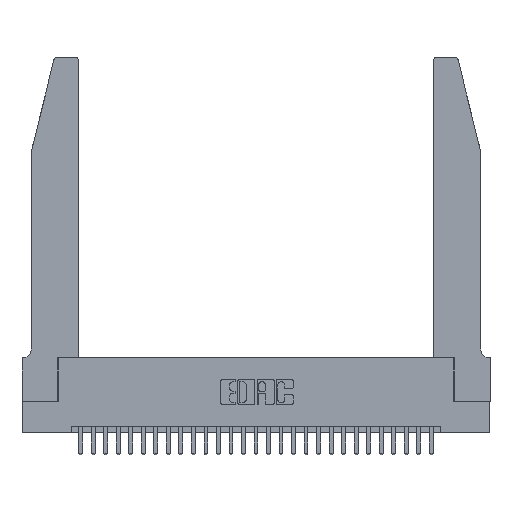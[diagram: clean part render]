
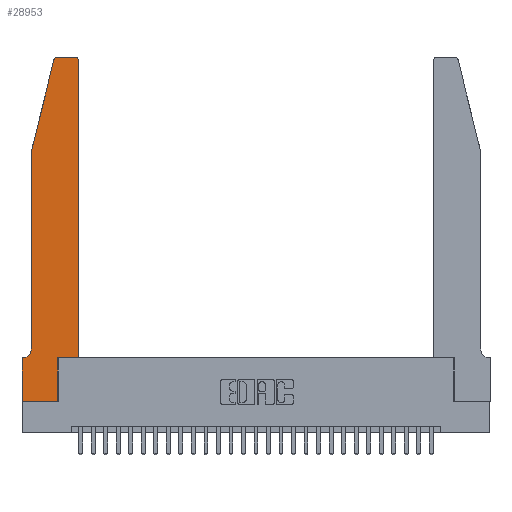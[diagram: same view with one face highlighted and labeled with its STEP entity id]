
A CAD part, top view. The second image highlights one B-rep face of the part: STEP entity #28953.
In plain terms, the highlighted planar face has unit normal (0, 0, 1).
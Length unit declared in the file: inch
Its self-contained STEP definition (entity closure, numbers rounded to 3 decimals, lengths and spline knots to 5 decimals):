
#121 = DIRECTION ( 'NONE',  ( 0., 0., 1. ) ) ;
#394 = VERTEX_POINT ( 'NONE', #3091 ) ;
#399 = ORIENTED_EDGE ( 'NONE', *, *, #19376, .T. ) ;
#493 = CARTESIAN_POINT ( 'NONE',  ( 0.0055, 0.42, 0.37 ) ) ;
#527 = EDGE_CURVE ( 'NONE', #394, #2790, #25859, .T. ) ;
#742 = LINE ( 'NONE', #20856, #5367 ) ;
#2523 = CARTESIAN_POINT ( 'NONE',  ( 0.284, 2.72, 0.37 ) ) ;
#2575 = CARTESIAN_POINT ( 'NONE',  ( 0.2865, 0.35, 0.37 ) ) ;
#2790 = VERTEX_POINT ( 'NONE', #20274 ) ;
#3091 = CARTESIAN_POINT ( 'NONE',  ( 0., 0.35, 0.37 ) ) ;
#3295 = VERTEX_POINT ( 'NONE', #20784 ) ;
#3761 = CARTESIAN_POINT ( 'NONE',  ( 0.4505, 0.35, 0.37 ) ) ;
#4062 = EDGE_CURVE ( 'NONE', #7007, #14862, #15695, .T. ) ;
#4589 = DIRECTION ( 'NONE',  ( 1., 0., 0. ) ) ;
#4986 = DIRECTION ( 'NONE',  ( -0.239, -0.971, 0. ) ) ;
#5217 = FACE_OUTER_BOUND ( 'NONE', #7160, .T. ) ;
#5367 = VECTOR ( 'NONE', #4986, 39.37008 ) ;
#5966 = DIRECTION ( 'NONE',  ( 0., 1., 0. ) ) ;
#6171 = DIRECTION ( 'NONE',  ( -1., 0., 0. ) ) ;
#7007 = VERTEX_POINT ( 'NONE', #2575 ) ;
#7160 = EDGE_LOOP ( 'NONE', ( #26678, #16221, #22059, #18440, #28837, #10267, #23125, #26511, #399, #26267, #19559, #9952 ) ) ;
#7229 = DIRECTION ( 'NONE',  ( 1., 0., 0. ) ) ;
#7350 = CIRCLE ( 'NONE', #19434, 0.07 ) ;
#7730 = VECTOR ( 'NONE', #8560, 39.37008 ) ;
#8003 = EDGE_CURVE ( 'NONE', #13516, #18174, #26152, .T. ) ;
#8112 = DIRECTION ( 'NONE',  ( 0., -1., 0. ) ) ;
#8218 = CARTESIAN_POINT ( 'NONE',  ( 0.4505, 2.72, 0.37 ) ) ;
#8560 = DIRECTION ( 'NONE',  ( 0., -1., 0. ) ) ;
#8812 = LINE ( 'NONE', #11809, #19114 ) ;
#9272 = PLANE ( 'NONE',  #11984 ) ;
#9444 = DIRECTION ( 'NONE',  ( 1., 0., 0. ) ) ;
#9820 = DIRECTION ( 'NONE',  ( 0., 0., -1. ) ) ;
#9952 = ORIENTED_EDGE ( 'NONE', *, *, #8003, .T. ) ;
#10073 = VERTEX_POINT ( 'NONE', #28441 ) ;
#10267 = ORIENTED_EDGE ( 'NONE', *, *, #28495, .T. ) ;
#10675 = AXIS2_PLACEMENT_3D ( 'NONE', #2523, #121, #4589 ) ;
#11598 = VECTOR ( 'NONE', #8112, 39.37008 ) ;
#11687 = DIRECTION ( 'NONE',  ( -1., 0., 0. ) ) ;
#11809 = CARTESIAN_POINT ( 'NONE',  ( 0., 0., 0.37 ) ) ;
#11901 = CARTESIAN_POINT ( 'NONE',  ( 0.4505, 0.35, 0.37 ) ) ;
#11984 = AXIS2_PLACEMENT_3D ( 'NONE', #19643, #15885, #15791 ) ;
#12388 = CARTESIAN_POINT ( 'NONE',  ( 0.0055, 0.35, 0.37 ) ) ;
#13315 = EDGE_CURVE ( 'NONE', #28248, #26819, #25479, .T. ) ;
#13516 = VERTEX_POINT ( 'NONE', #8218 ) ;
#14143 = AXIS2_PLACEMENT_3D ( 'NONE', #16209, #18530, #7229 ) ;
#14535 = CIRCLE ( 'NONE', #10675, 0.03 ) ;
#14862 = VERTEX_POINT ( 'NONE', #3761 ) ;
#14934 = EDGE_CURVE ( 'NONE', #18174, #10073, #28572, .T. ) ;
#15695 = LINE ( 'NONE', #11901, #17860 ) ;
#15791 = DIRECTION ( 'NONE',  ( 1., 0., 0. ) ) ;
#15844 = VECTOR ( 'NONE', #19221, 39.37008 ) ;
#15885 = DIRECTION ( 'NONE',  ( 0., 0., 1. ) ) ;
#16209 = CARTESIAN_POINT ( 'NONE',  ( 0.4205, 2.72, 0.37 ) ) ;
#16221 = ORIENTED_EDGE ( 'NONE', *, *, #16845, .T. ) ;
#16845 = EDGE_CURVE ( 'NONE', #10073, #21601, #14535, .T. ) ;
#16927 = EDGE_CURVE ( 'NONE', #21601, #28248, #742, .T. ) ;
#17142 = CARTESIAN_POINT ( 'NONE',  ( 0.25487, 2.72718, 0.37 ) ) ;
#17145 = CARTESIAN_POINT ( 'NONE',  ( 0.2865, 0.35, 0.37 ) ) ;
#17860 = VECTOR ( 'NONE', #19080, 39.37008 ) ;
#18013 = LINE ( 'NONE', #28066, #15844 ) ;
#18174 = VERTEX_POINT ( 'NONE', #21461 ) ;
#18440 = ORIENTED_EDGE ( 'NONE', *, *, #13315, .T. ) ;
#18530 = DIRECTION ( 'NONE',  ( 0., 0., 1. ) ) ;
#19080 = DIRECTION ( 'NONE',  ( 1., 0., 0. ) ) ;
#19114 = VECTOR ( 'NONE', #9444, 39.37008 ) ;
#19137 = EDGE_CURVE ( 'NONE', #2790, #3295, #8812, .T. ) ;
#19221 = DIRECTION ( 'NONE',  ( -1., 0., 0. ) ) ;
#19376 = EDGE_CURVE ( 'NONE', #3295, #7007, #25132, .T. ) ;
#19434 = AXIS2_PLACEMENT_3D ( 'NONE', #493, #9820, #11687 ) ;
#19447 = CARTESIAN_POINT ( 'NONE',  ( 0.2605, 2.75, 0.37 ) ) ;
#19559 = ORIENTED_EDGE ( 'NONE', *, *, #24553, .T. ) ;
#19641 = EDGE_CURVE ( 'NONE', #26819, #22756, #7350, .T. ) ;
#19643 = CARTESIAN_POINT ( 'NONE',  ( 0., 0.35, 0.37 ) ) ;
#20254 = CARTESIAN_POINT ( 'NONE',  ( 0., 0., 0.37 ) ) ;
#20274 = CARTESIAN_POINT ( 'NONE',  ( 0., 0., 0.37 ) ) ;
#20323 = CARTESIAN_POINT ( 'NONE',  ( 0.4505, 0.35, 0.37 ) ) ;
#20784 = CARTESIAN_POINT ( 'NONE',  ( 0.2865, 0., 0.37 ) ) ;
#20856 = CARTESIAN_POINT ( 'NONE',  ( 0.0755, 2., 0.37 ) ) ;
#21461 = CARTESIAN_POINT ( 'NONE',  ( 0.4205, 2.75, 0.37 ) ) ;
#21601 = VERTEX_POINT ( 'NONE', #17142 ) ;
#22059 = ORIENTED_EDGE ( 'NONE', *, *, #16927, .T. ) ;
#22681 = VECTOR ( 'NONE', #5966, 39.37008 ) ;
#22756 = VERTEX_POINT ( 'NONE', #12388 ) ;
#23125 = ORIENTED_EDGE ( 'NONE', *, *, #527, .T. ) ;
#23334 = CARTESIAN_POINT ( 'NONE',  ( 0.0755, 2., 0.37 ) ) ;
#24553 = EDGE_CURVE ( 'NONE', #14862, #13516, #25570, .T. ) ;
#24604 = CARTESIAN_POINT ( 'NONE',  ( 0.0755, 0.42, 0.37 ) ) ;
#25004 = DIRECTION ( 'NONE',  ( 0., 1., 0. ) ) ;
#25113 = CARTESIAN_POINT ( 'NONE',  ( 0.0755, 2., 0.37 ) ) ;
#25132 = LINE ( 'NONE', #17145, #22681 ) ;
#25199 = VECTOR ( 'NONE', #25004, 39.37008 ) ;
#25479 = LINE ( 'NONE', #23334, #11598 ) ;
#25570 = LINE ( 'NONE', #20323, #25199 ) ;
#25859 = LINE ( 'NONE', #20254, #7730 ) ;
#26152 = CIRCLE ( 'NONE', #14143, 0.03 ) ;
#26267 = ORIENTED_EDGE ( 'NONE', *, *, #4062, .T. ) ;
#26511 = ORIENTED_EDGE ( 'NONE', *, *, #19137, .T. ) ;
#26678 = ORIENTED_EDGE ( 'NONE', *, *, #14934, .T. ) ;
#26819 = VERTEX_POINT ( 'NONE', #24604 ) ;
#27141 = VECTOR ( 'NONE', #6171, 39.37008 ) ;
#28066 = CARTESIAN_POINT ( 'NONE',  ( 0.0755, 0.35, 0.37 ) ) ;
#28248 = VERTEX_POINT ( 'NONE', #25113 ) ;
#28441 = CARTESIAN_POINT ( 'NONE',  ( 0.284, 2.75, 0.37 ) ) ;
#28495 = EDGE_CURVE ( 'NONE', #22756, #394, #18013, .T. ) ;
#28572 = LINE ( 'NONE', #19447, #27141 ) ;
#28837 = ORIENTED_EDGE ( 'NONE', *, *, #19641, .T. ) ;
#28953 = ADVANCED_FACE ( 'NONE', ( #5217 ), #9272, .T. ) ;
